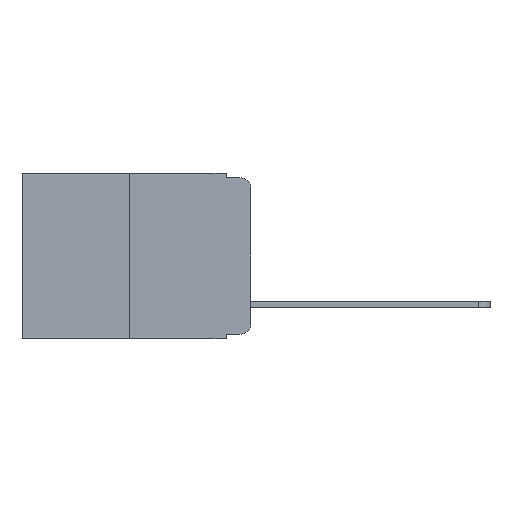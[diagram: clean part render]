
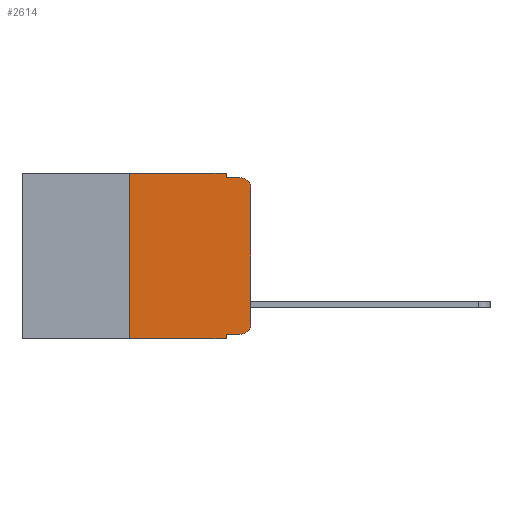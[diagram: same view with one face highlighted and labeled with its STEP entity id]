
A CAD part, left-side view. The second image highlights one B-rep face of the part: STEP entity #2614.
In plain terms, the highlighted planar face has unit normal (-1, 0, 0).
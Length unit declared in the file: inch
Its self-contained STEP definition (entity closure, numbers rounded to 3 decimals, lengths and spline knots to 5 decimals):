
#838 = LINE ( 'NONE', #19196, #18118 ) ;
#1046 = LINE ( 'NONE', #8180, #5700 ) ;
#1195 = VERTEX_POINT ( 'NONE', #13479 ) ;
#1276 = EDGE_CURVE ( 'NONE', #14005, #14908, #9572, .T. ) ;
#1394 = EDGE_CURVE ( 'NONE', #20973, #21087, #13477, .T. ) ;
#2518 = FACE_OUTER_BOUND ( 'NONE', #14770, .T. ) ;
#2614 = ADVANCED_FACE ( 'NONE', ( #2518 ), #8073, .F. ) ;
#2808 = AXIS2_PLACEMENT_3D ( 'NONE', #20975, #12659, #20864 ) ;
#3248 = DIRECTION ( 'NONE',  ( -1., 0., 0. ) ) ;
#3369 = CARTESIAN_POINT ( 'NONE',  ( 0., 0.02, -0.01 ) ) ;
#3716 = VECTOR ( 'NONE', #20161, 39.37008 ) ;
#3918 = CARTESIAN_POINT ( 'NONE',  ( 0., 0.02, -0.03 ) ) ;
#3976 = CARTESIAN_POINT ( 'NONE',  ( 0., 0.02, -0.313 ) ) ;
#4273 = VERTEX_POINT ( 'NONE', #13384 ) ;
#4839 = VERTEX_POINT ( 'NONE', #14500 ) ;
#5330 = LINE ( 'NONE', #20857, #17925 ) ;
#5700 = VECTOR ( 'NONE', #16074, 39.37008 ) ;
#5816 = DIRECTION ( 'NONE',  ( 0., 0., -1. ) ) ;
#6131 = EDGE_CURVE ( 'NONE', #4273, #14005, #15668, .T. ) ;
#6757 = LINE ( 'NONE', #19060, #13767 ) ;
#7164 = CARTESIAN_POINT ( 'NONE',  ( 0., 0., -0.313 ) ) ;
#7314 = VECTOR ( 'NONE', #18367, 39.37008 ) ;
#7422 = LINE ( 'NONE', #18855, #10759 ) ;
#8073 = PLANE ( 'NONE',  #2808 ) ;
#8180 = CARTESIAN_POINT ( 'NONE',  ( 0., 0.051, 0. ) ) ;
#8271 = CARTESIAN_POINT ( 'NONE',  ( 0., 0.473, 0. ) ) ;
#8425 = LINE ( 'NONE', #9686, #3716 ) ;
#8794 = CARTESIAN_POINT ( 'NONE',  ( 0., 0.051, 0. ) ) ;
#9572 = LINE ( 'NONE', #8271, #13225 ) ;
#9686 = CARTESIAN_POINT ( 'NONE',  ( 0., 0., 0. ) ) ;
#9964 = DIRECTION ( 'NONE',  ( 0., -1., 0. ) ) ;
#10759 = VECTOR ( 'NONE', #12861, 39.37008 ) ;
#10826 = VERTEX_POINT ( 'NONE', #3369 ) ;
#10939 = EDGE_CURVE ( 'NONE', #12213, #20973, #5330, .T. ) ;
#11602 = EDGE_CURVE ( 'NONE', #14908, #15813, #7422, .T. ) ;
#11840 = CARTESIAN_POINT ( 'NONE',  ( 0., 0.02, -0.333 ) ) ;
#12034 = ORIENTED_EDGE ( 'NONE', *, *, #17333, .T. ) ;
#12213 = VERTEX_POINT ( 'NONE', #19864 ) ;
#12618 = EDGE_CURVE ( 'NONE', #15813, #10826, #838, .T. ) ;
#12659 = DIRECTION ( 'NONE',  ( 1., 0., 0. ) ) ;
#12728 = ORIENTED_EDGE ( 'NONE', *, *, #13662, .T. ) ;
#12861 = DIRECTION ( 'NONE',  ( 0., 0., -1. ) ) ;
#12965 = ORIENTED_EDGE ( 'NONE', *, *, #12618, .F. ) ;
#13170 = DIRECTION ( 'NONE',  ( 0., -1., 0. ) ) ;
#13225 = VECTOR ( 'NONE', #19193, 39.37008 ) ;
#13384 = CARTESIAN_POINT ( 'NONE',  ( 0., 0.25, -0.343 ) ) ;
#13477 = CIRCLE ( 'NONE', #19358, 0.02 ) ;
#13479 = CARTESIAN_POINT ( 'NONE',  ( 0., 0., -0.03 ) ) ;
#13507 = DIRECTION ( 'NONE',  ( 0., -1., 0. ) ) ;
#13662 = EDGE_CURVE ( 'NONE', #1195, #10826, #17408, .T. ) ;
#13767 = VECTOR ( 'NONE', #9964, 39.37008 ) ;
#14005 = VERTEX_POINT ( 'NONE', #18790 ) ;
#14149 = CARTESIAN_POINT ( 'NONE',  ( 0., 0.051, -0.01 ) ) ;
#14185 = ORIENTED_EDGE ( 'NONE', *, *, #11602, .F. ) ;
#14500 = CARTESIAN_POINT ( 'NONE',  ( 0., 0.051, -0.343 ) ) ;
#14682 = ORIENTED_EDGE ( 'NONE', *, *, #1276, .F. ) ;
#14752 = ORIENTED_EDGE ( 'NONE', *, *, #6131, .F. ) ;
#14770 = EDGE_LOOP ( 'NONE', ( #12034, #12728, #12965, #14185, #14682, #14752, #16778, #16801, #16856, #17652 ) ) ;
#14908 = VERTEX_POINT ( 'NONE', #8794 ) ;
#15326 = DIRECTION ( 'NONE',  ( -1., 0., 0. ) ) ;
#15572 = AXIS2_PLACEMENT_3D ( 'NONE', #3918, #15326, #5816 ) ;
#15668 = LINE ( 'NONE', #18364, #7314 ) ;
#15813 = VERTEX_POINT ( 'NONE', #14149 ) ;
#16074 = DIRECTION ( 'NONE',  ( 0., 0., -1. ) ) ;
#16778 = ORIENTED_EDGE ( 'NONE', *, *, #20004, .T. ) ;
#16801 = ORIENTED_EDGE ( 'NONE', *, *, #19967, .F. ) ;
#16837 = DIRECTION ( 'NONE',  ( 0., 0., -1. ) ) ;
#16856 = ORIENTED_EDGE ( 'NONE', *, *, #10939, .T. ) ;
#17333 = EDGE_CURVE ( 'NONE', #21087, #1195, #8425, .T. ) ;
#17408 = CIRCLE ( 'NONE', #15572, 0.02 ) ;
#17652 = ORIENTED_EDGE ( 'NONE', *, *, #1394, .T. ) ;
#17925 = VECTOR ( 'NONE', #13507, 39.37008 ) ;
#18118 = VECTOR ( 'NONE', #13170, 39.37008 ) ;
#18364 = CARTESIAN_POINT ( 'NONE',  ( 0., 0.25, 0. ) ) ;
#18367 = DIRECTION ( 'NONE',  ( 0., 0., 1. ) ) ;
#18790 = CARTESIAN_POINT ( 'NONE',  ( 0., 0.25, 0. ) ) ;
#18855 = CARTESIAN_POINT ( 'NONE',  ( 0., 0.051, 0. ) ) ;
#19060 = CARTESIAN_POINT ( 'NONE',  ( 0., 0.473, -0.343 ) ) ;
#19193 = DIRECTION ( 'NONE',  ( 0., -1., 0. ) ) ;
#19196 = CARTESIAN_POINT ( 'NONE',  ( 0., 0.051, -0.01 ) ) ;
#19358 = AXIS2_PLACEMENT_3D ( 'NONE', #3976, #3248, #16837 ) ;
#19864 = CARTESIAN_POINT ( 'NONE',  ( 0., 0.051, -0.333 ) ) ;
#19967 = EDGE_CURVE ( 'NONE', #12213, #4839, #1046, .T. ) ;
#20004 = EDGE_CURVE ( 'NONE', #4273, #4839, #6757, .T. ) ;
#20161 = DIRECTION ( 'NONE',  ( 0., 0., 1. ) ) ;
#20857 = CARTESIAN_POINT ( 'NONE',  ( 0., 0.051, -0.333 ) ) ;
#20864 = DIRECTION ( 'NONE',  ( 0., 0., -1. ) ) ;
#20973 = VERTEX_POINT ( 'NONE', #11840 ) ;
#20975 = CARTESIAN_POINT ( 'NONE',  ( 0., 0.473, 0. ) ) ;
#21087 = VERTEX_POINT ( 'NONE', #7164 ) ;
